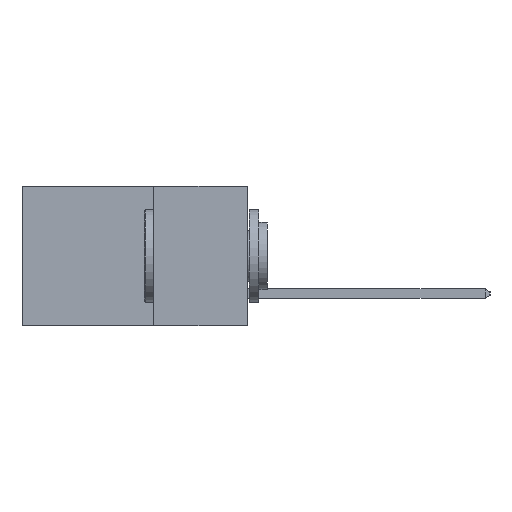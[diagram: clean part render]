
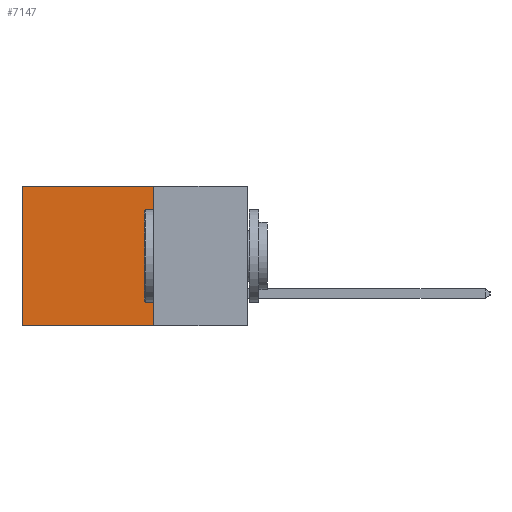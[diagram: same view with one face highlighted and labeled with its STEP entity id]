
A CAD part, left-side view. The second image highlights one B-rep face of the part: STEP entity #7147.
In plain terms, the highlighted planar face has unit normal (-1, 0, 0).
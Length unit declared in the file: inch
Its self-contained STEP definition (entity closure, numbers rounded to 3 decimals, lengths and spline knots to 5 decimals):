
#1950 = CARTESIAN_POINT ( 'NONE',  ( 0.2615, 0.25, 0. ) ) ;
#2192 = VECTOR ( 'NONE', #19851, 39.37008 ) ;
#2593 = ORIENTED_EDGE ( 'NONE', *, *, #14344, .T. ) ;
#2658 = LINE ( 'NONE', #19888, #2192 ) ;
#2853 = ORIENTED_EDGE ( 'NONE', *, *, #6052, .F. ) ;
#3338 = FACE_OUTER_BOUND ( 'NONE', #10029, .T. ) ;
#3348 = LINE ( 'NONE', #18700, #11398 ) ;
#3504 = EDGE_CURVE ( 'NONE', #15420, #6376, #17531, .T. ) ;
#3838 = LINE ( 'NONE', #10131, #8102 ) ;
#6052 = EDGE_CURVE ( 'NONE', #10528, #15420, #2658, .T. ) ;
#6376 = VERTEX_POINT ( 'NONE', #16922 ) ;
#6969 = CARTESIAN_POINT ( 'NONE',  ( 0.2615, 0.25, -0.37 ) ) ;
#7044 = VERTEX_POINT ( 'NONE', #10305 ) ;
#7147 = ADVANCED_FACE ( 'NONE', ( #3338 ), #9291, .F. ) ;
#8102 = VECTOR ( 'NONE', #10075, 39.37008 ) ;
#8783 = EDGE_CURVE ( 'NONE', #7044, #6376, #3838, .T. ) ;
#8792 = DIRECTION ( 'NONE',  ( 0., 0., -1. ) ) ;
#8814 = DIRECTION ( 'NONE',  ( 1., 0., 0. ) ) ;
#8973 = VECTOR ( 'NONE', #18802, 39.37008 ) ;
#9025 = CARTESIAN_POINT ( 'NONE',  ( 0.2615, 0.25, -0.37 ) ) ;
#9291 = PLANE ( 'NONE',  #11499 ) ;
#10029 = EDGE_LOOP ( 'NONE', ( #16714, #20473, #2853, #2593 ) ) ;
#10075 = DIRECTION ( 'NONE',  ( 0., 0., -1. ) ) ;
#10131 = CARTESIAN_POINT ( 'NONE',  ( 0.2615, 0.6, -0.37 ) ) ;
#10305 = CARTESIAN_POINT ( 'NONE',  ( 0.2615, 0.6, 0. ) ) ;
#10528 = VERTEX_POINT ( 'NONE', #1950 ) ;
#11398 = VECTOR ( 'NONE', #14038, 39.37008 ) ;
#11499 = AXIS2_PLACEMENT_3D ( 'NONE', #9025, #8814, #8792 ) ;
#14038 = DIRECTION ( 'NONE',  ( 0., 1., 0. ) ) ;
#14344 = EDGE_CURVE ( 'NONE', #10528, #7044, #3348, .T. ) ;
#15420 = VERTEX_POINT ( 'NONE', #16116 ) ;
#16116 = CARTESIAN_POINT ( 'NONE',  ( 0.2615, 0.25, -0.37 ) ) ;
#16714 = ORIENTED_EDGE ( 'NONE', *, *, #8783, .T. ) ;
#16922 = CARTESIAN_POINT ( 'NONE',  ( 0.2615, 0.6, -0.37 ) ) ;
#17531 = LINE ( 'NONE', #6969, #8973 ) ;
#18700 = CARTESIAN_POINT ( 'NONE',  ( 0.2615, 0.25, 0. ) ) ;
#18802 = DIRECTION ( 'NONE',  ( 0., 1., 0. ) ) ;
#19851 = DIRECTION ( 'NONE',  ( 0., 0., -1. ) ) ;
#19888 = CARTESIAN_POINT ( 'NONE',  ( 0.2615, 0.25, -0.37 ) ) ;
#20473 = ORIENTED_EDGE ( 'NONE', *, *, #3504, .F. ) ;
